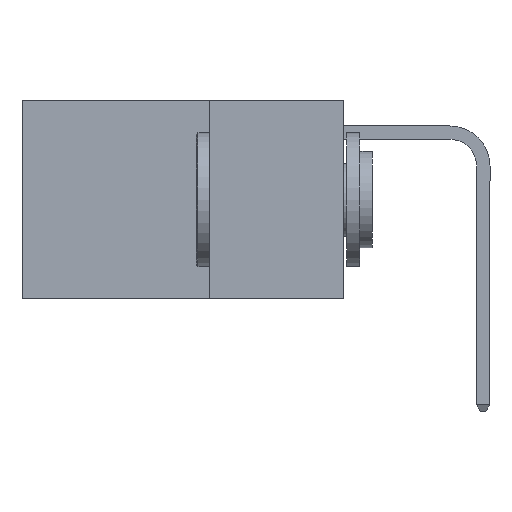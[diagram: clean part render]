
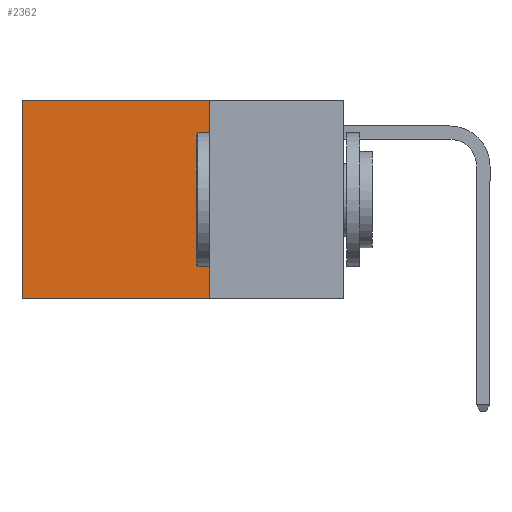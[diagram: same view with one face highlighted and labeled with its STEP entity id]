
A CAD part, left-side view. The second image highlights one B-rep face of the part: STEP entity #2362.
In plain terms, the highlighted planar face has unit normal (-1, 0, 0).
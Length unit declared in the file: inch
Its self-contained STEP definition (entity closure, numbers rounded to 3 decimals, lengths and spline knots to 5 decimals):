
#145 = DIRECTION ( 'NONE',  ( 0., 1., 0. ) ) ;
#574 = CARTESIAN_POINT ( 'NONE',  ( 0.2625, 0.6, -0.37 ) ) ;
#726 = ORIENTED_EDGE ( 'NONE', *, *, #7272, .T. ) ;
#968 = CARTESIAN_POINT ( 'NONE',  ( 0.2625, 0.25, -0.37 ) ) ;
#1182 = CARTESIAN_POINT ( 'NONE',  ( 0.2625, 0.25, 0. ) ) ;
#1422 = VECTOR ( 'NONE', #145, 39.37008 ) ;
#2073 = EDGE_LOOP ( 'NONE', ( #726, #11849, #4902, #10076 ) ) ;
#2362 = ADVANCED_FACE ( 'NONE', ( #4090 ), #11888, .F. ) ;
#2649 = DIRECTION ( 'NONE',  ( 0., 0., -1. ) ) ;
#2781 = VERTEX_POINT ( 'NONE', #574 ) ;
#4090 = FACE_OUTER_BOUND ( 'NONE', #2073, .T. ) ;
#4357 = VERTEX_POINT ( 'NONE', #8135 ) ;
#4381 = DIRECTION ( 'NONE',  ( 0., 1., 0. ) ) ;
#4824 = VECTOR ( 'NONE', #2649, 39.37008 ) ;
#4902 = ORIENTED_EDGE ( 'NONE', *, *, #9966, .F. ) ;
#5012 = LINE ( 'NONE', #11532, #9620 ) ;
#5150 = VECTOR ( 'NONE', #4381, 39.37008 ) ;
#5455 = CARTESIAN_POINT ( 'NONE',  ( 0.2625, 0.25, 0. ) ) ;
#6749 = EDGE_CURVE ( 'NONE', #8194, #2781, #9489, .T. ) ;
#7019 = CARTESIAN_POINT ( 'NONE',  ( 0.2625, 0.6, 0. ) ) ;
#7272 = EDGE_CURVE ( 'NONE', #9562, #2781, #5012, .T. ) ;
#8135 = CARTESIAN_POINT ( 'NONE',  ( 0.2625, 0.25, 0. ) ) ;
#8194 = VERTEX_POINT ( 'NONE', #968 ) ;
#8310 = EDGE_CURVE ( 'NONE', #4357, #9562, #11444, .T. ) ;
#8349 = CARTESIAN_POINT ( 'NONE',  ( 0.2625, 0.25, 0. ) ) ;
#8880 = DIRECTION ( 'NONE',  ( 0., 0., -1. ) ) ;
#9146 = LINE ( 'NONE', #8349, #4824 ) ;
#9489 = LINE ( 'NONE', #9894, #5150 ) ;
#9562 = VERTEX_POINT ( 'NONE', #7019 ) ;
#9620 = VECTOR ( 'NONE', #8880, 39.37008 ) ;
#9894 = CARTESIAN_POINT ( 'NONE',  ( 0.2625, 0.25, -0.37 ) ) ;
#9966 = EDGE_CURVE ( 'NONE', #4357, #8194, #9146, .T. ) ;
#10076 = ORIENTED_EDGE ( 'NONE', *, *, #8310, .T. ) ;
#10131 = AXIS2_PLACEMENT_3D ( 'NONE', #5455, #11902, #12071 ) ;
#11444 = LINE ( 'NONE', #1182, #1422 ) ;
#11532 = CARTESIAN_POINT ( 'NONE',  ( 0.2625, 0.6, 0. ) ) ;
#11849 = ORIENTED_EDGE ( 'NONE', *, *, #6749, .F. ) ;
#11888 = PLANE ( 'NONE',  #10131 ) ;
#11902 = DIRECTION ( 'NONE',  ( 1., 0., 0. ) ) ;
#12071 = DIRECTION ( 'NONE',  ( 0., 0., -1. ) ) ;
